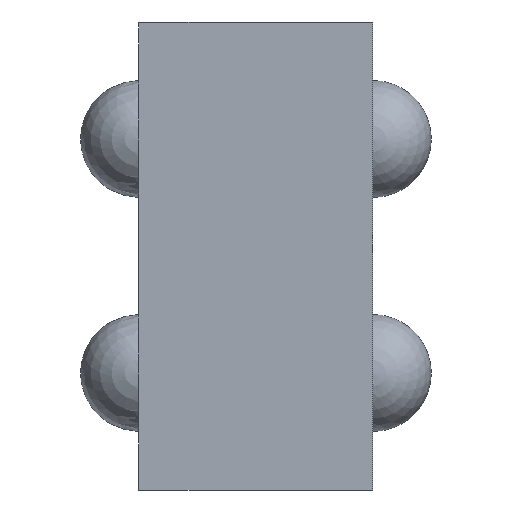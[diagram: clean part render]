
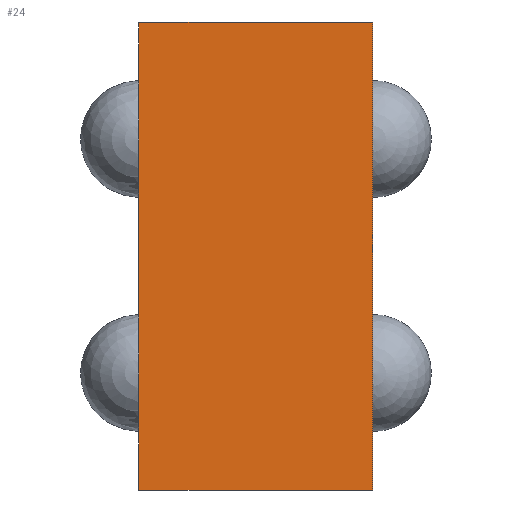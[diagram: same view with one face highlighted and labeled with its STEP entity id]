
A CAD part, front view. The second image highlights one B-rep face of the part: STEP entity #24.
In plain terms, the highlighted planar face has unit normal (0, -1, 0).
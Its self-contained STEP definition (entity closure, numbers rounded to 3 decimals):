
#3 = CARTESIAN_POINT ( 'NONE',  ( 0., -5., 10. ) ) ;
#10 = EDGE_CURVE ( 'NONE', #285, #242, #246, .T. ) ;
#14 = DIRECTION ( 'NONE',  ( 0., 0., -1. ) ) ;
#17 = PLANE ( 'NONE',  #363 ) ;
#24 = ADVANCED_FACE ( 'NONE', ( #215 ), #17, .F. ) ;
#29 = EDGE_CURVE ( 'NONE', #318, #339, #207, .T. ) ;
#37 = EDGE_CURVE ( 'NONE', #318, #285, #206, .T. ) ;
#41 = CARTESIAN_POINT ( 'NONE',  ( 0., -5., -10. ) ) ;
#56 = VECTOR ( 'NONE', #271, 1000. ) ;
#61 = LINE ( 'NONE', #41, #56 ) ;
#63 = DIRECTION ( 'NONE',  ( -1., 0., 0. ) ) ;
#92 = DIRECTION ( 'NONE',  ( -1., 0., 0. ) ) ;
#146 = CARTESIAN_POINT ( 'NONE',  ( 10., -5., -10. ) ) ;
#149 = CARTESIAN_POINT ( 'NONE',  ( 10., -5., 10. ) ) ;
#165 = CARTESIAN_POINT ( 'NONE',  ( 10., -5., -10. ) ) ;
#194 = VECTOR ( 'NONE', #14, 1000. ) ;
#203 = DIRECTION ( 'NONE',  ( 0., 0., 1. ) ) ;
#206 = LINE ( 'NONE', #418, #194 ) ;
#207 = LINE ( 'NONE', #275, #227 ) ;
#215 = FACE_OUTER_BOUND ( 'NONE', #322, .T. ) ;
#219 = VECTOR ( 'NONE', #92, 1000. ) ;
#227 = VECTOR ( 'NONE', #63, 1000. ) ;
#242 = VERTEX_POINT ( 'NONE', #399 ) ;
#246 = LINE ( 'NONE', #335, #219 ) ;
#257 = ORIENTED_EDGE ( 'NONE', *, *, #411, .T. ) ;
#271 = DIRECTION ( 'NONE',  ( 0., 0., -1. ) ) ;
#275 = CARTESIAN_POINT ( 'NONE',  ( 10., -5., 10. ) ) ;
#285 = VERTEX_POINT ( 'NONE', #146 ) ;
#318 = VERTEX_POINT ( 'NONE', #149 ) ;
#322 = EDGE_LOOP ( 'NONE', ( #257, #376, #417, #359 ) ) ;
#335 = CARTESIAN_POINT ( 'NONE',  ( 10., -5., -10. ) ) ;
#339 = VERTEX_POINT ( 'NONE', #3 ) ;
#359 = ORIENTED_EDGE ( 'NONE', *, *, #29, .T. ) ;
#363 = AXIS2_PLACEMENT_3D ( 'NONE', #165, #416, #203 ) ;
#376 = ORIENTED_EDGE ( 'NONE', *, *, #10, .F. ) ;
#399 = CARTESIAN_POINT ( 'NONE',  ( 0., -5., -10. ) ) ;
#411 = EDGE_CURVE ( 'NONE', #339, #242, #61, .T. ) ;
#416 = DIRECTION ( 'NONE',  ( 0., 1., 0. ) ) ;
#417 = ORIENTED_EDGE ( 'NONE', *, *, #37, .F. ) ;
#418 = CARTESIAN_POINT ( 'NONE',  ( 10., -5., -10. ) ) ;
